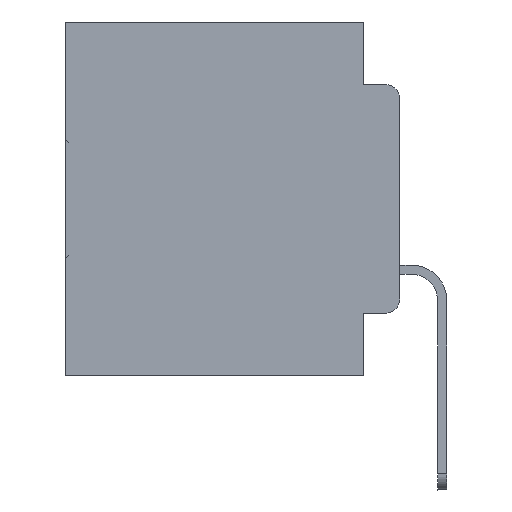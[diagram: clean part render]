
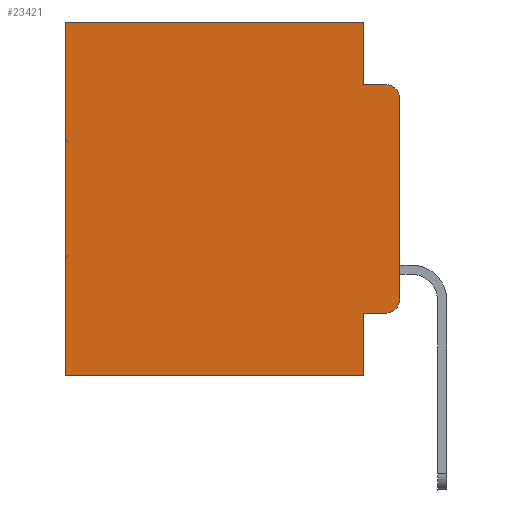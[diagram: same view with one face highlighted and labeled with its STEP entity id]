
A CAD part, left-side view. The second image highlights one B-rep face of the part: STEP entity #23421.
In plain terms, the highlighted planar face has unit normal (-1, 0, 0).
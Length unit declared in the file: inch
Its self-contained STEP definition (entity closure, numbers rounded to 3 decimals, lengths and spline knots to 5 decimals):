
#5 = DIRECTION ( 'NONE',  ( 1., 0., 0. ) ) ;
#20 = EDGE_CURVE ( 'NONE', #6397, #1886, #21172, .T. ) ;
#800 = CARTESIAN_POINT ( 'NONE',  ( 0.298, 0.473, 0. ) ) ;
#909 = VERTEX_POINT ( 'NONE', #26508 ) ;
#1021 = CIRCLE ( 'NONE', #22861, 0.02 ) ;
#1120 = CARTESIAN_POINT ( 'NONE',  ( 0.298, 0.051, -0.4115 ) ) ;
#1125 = VERTEX_POINT ( 'NONE', #22896 ) ;
#1173 = CARTESIAN_POINT ( 'NONE',  ( 0.298, 0.051, 0. ) ) ;
#1886 = VERTEX_POINT ( 'NONE', #12720 ) ;
#1897 = CARTESIAN_POINT ( 'NONE',  ( 0.298, 0.051, -0.0885 ) ) ;
#2144 = AXIS2_PLACEMENT_3D ( 'NONE', #3751, #5, #31906 ) ;
#2297 = DIRECTION ( 'NONE',  ( 0., 0., -1. ) ) ;
#2820 = EDGE_CURVE ( 'NONE', #12477, #6620, #18144, .T. ) ;
#2948 = VERTEX_POINT ( 'NONE', #6425 ) ;
#3010 = CARTESIAN_POINT ( 'NONE',  ( 0.298, 0.051, 0. ) ) ;
#3590 = FACE_OUTER_BOUND ( 'NONE', #11234, .T. ) ;
#3751 = CARTESIAN_POINT ( 'NONE',  ( 0.298, 0., 0. ) ) ;
#4427 = CARTESIAN_POINT ( 'NONE',  ( 0.298, 0.051, 0. ) ) ;
#4510 = ORIENTED_EDGE ( 'NONE', *, *, #13917, .T. ) ;
#5622 = ORIENTED_EDGE ( 'NONE', *, *, #18519, .F. ) ;
#5911 = DIRECTION ( 'NONE',  ( 0., 0., -1. ) ) ;
#6081 = ORIENTED_EDGE ( 'NONE', *, *, #21125, .F. ) ;
#6397 = VERTEX_POINT ( 'NONE', #4427 ) ;
#6425 = CARTESIAN_POINT ( 'NONE',  ( 0.298, 0.473, -0.5 ) ) ;
#6620 = VERTEX_POINT ( 'NONE', #25820 ) ;
#6802 = VECTOR ( 'NONE', #19143, 39.37008 ) ;
#7545 = VECTOR ( 'NONE', #28842, 39.37008 ) ;
#8650 = CARTESIAN_POINT ( 'NONE',  ( 0.298, 0., 0. ) ) ;
#8699 = VECTOR ( 'NONE', #30675, 39.37008 ) ;
#9064 = LINE ( 'NONE', #1897, #6802 ) ;
#9298 = CARTESIAN_POINT ( 'NONE',  ( 0.298, 0., -0.5 ) ) ;
#10515 = DIRECTION ( 'NONE',  ( 0., 0., -1. ) ) ;
#10802 = CARTESIAN_POINT ( 'NONE',  ( 0.298, 0.02, -0.3915 ) ) ;
#11234 = EDGE_LOOP ( 'NONE', ( #30534, #20352, #5622, #6081, #18322, #4510, #27041, #26070, #20592, #11440 ) ) ;
#11243 = EDGE_CURVE ( 'NONE', #18020, #28091, #24690, .T. ) ;
#11393 = CARTESIAN_POINT ( 'NONE',  ( 0.298, 0.02, -0.4115 ) ) ;
#11440 = ORIENTED_EDGE ( 'NONE', *, *, #11837, .T. ) ;
#11691 = VECTOR ( 'NONE', #19012, 39.37008 ) ;
#11837 = EDGE_CURVE ( 'NONE', #28091, #6620, #18080, .T. ) ;
#11838 = CARTESIAN_POINT ( 'NONE',  ( 0.298, 0.051, -0.4115 ) ) ;
#11879 = VERTEX_POINT ( 'NONE', #25911 ) ;
#12144 = VECTOR ( 'NONE', #10515, 39.37008 ) ;
#12477 = VERTEX_POINT ( 'NONE', #21923 ) ;
#12698 = LINE ( 'NONE', #800, #22877 ) ;
#12720 = CARTESIAN_POINT ( 'NONE',  ( 0.298, 0.473, 0. ) ) ;
#13520 = PLANE ( 'NONE',  #2144 ) ;
#13917 = EDGE_CURVE ( 'NONE', #1886, #2948, #12698, .T. ) ;
#14033 = LINE ( 'NONE', #9298, #14795 ) ;
#14795 = VECTOR ( 'NONE', #29005, 39.37008 ) ;
#15482 = AXIS2_PLACEMENT_3D ( 'NONE', #10802, #18277, #5911 ) ;
#17260 = CARTESIAN_POINT ( 'NONE',  ( 0.298, 0.02, -0.1085 ) ) ;
#17596 = EDGE_CURVE ( 'NONE', #12477, #11879, #1021, .T. ) ;
#17700 = VECTOR ( 'NONE', #28203, 39.37008 ) ;
#18020 = VERTEX_POINT ( 'NONE', #1120 ) ;
#18080 = CIRCLE ( 'NONE', #15482, 0.02 ) ;
#18144 = LINE ( 'NONE', #25629, #8699 ) ;
#18268 = LINE ( 'NONE', #1173, #17700 ) ;
#18277 = DIRECTION ( 'NONE',  ( -1., 0., 0. ) ) ;
#18322 = ORIENTED_EDGE ( 'NONE', *, *, #20, .T. ) ;
#18519 = EDGE_CURVE ( 'NONE', #1125, #11879, #9064, .T. ) ;
#19012 = DIRECTION ( 'NONE',  ( 0., -1., 0. ) ) ;
#19143 = DIRECTION ( 'NONE',  ( 0., -1., 0. ) ) ;
#19222 = DIRECTION ( 'NONE',  ( -1., 0., 0. ) ) ;
#20352 = ORIENTED_EDGE ( 'NONE', *, *, #17596, .T. ) ;
#20592 = ORIENTED_EDGE ( 'NONE', *, *, #11243, .T. ) ;
#21125 = EDGE_CURVE ( 'NONE', #6397, #1125, #25325, .T. ) ;
#21172 = LINE ( 'NONE', #8650, #7545 ) ;
#21923 = CARTESIAN_POINT ( 'NONE',  ( 0.298, 0., -0.1085 ) ) ;
#22861 = AXIS2_PLACEMENT_3D ( 'NONE', #17260, #19222, #2297 ) ;
#22877 = VECTOR ( 'NONE', #22922, 39.37008 ) ;
#22896 = CARTESIAN_POINT ( 'NONE',  ( 0.298, 0.051, -0.0885 ) ) ;
#22922 = DIRECTION ( 'NONE',  ( 0., 0., -1. ) ) ;
#23421 = ADVANCED_FACE ( 'NONE', ( #3590 ), #13520, .F. ) ;
#24690 = LINE ( 'NONE', #11838, #11691 ) ;
#25325 = LINE ( 'NONE', #3010, #12144 ) ;
#25629 = CARTESIAN_POINT ( 'NONE',  ( 0.298, 0., 0. ) ) ;
#25820 = CARTESIAN_POINT ( 'NONE',  ( 0.298, 0., -0.3915 ) ) ;
#25911 = CARTESIAN_POINT ( 'NONE',  ( 0.298, 0.02, -0.0885 ) ) ;
#26070 = ORIENTED_EDGE ( 'NONE', *, *, #28660, .F. ) ;
#26508 = CARTESIAN_POINT ( 'NONE',  ( 0.298, 0.051, -0.5 ) ) ;
#26654 = EDGE_CURVE ( 'NONE', #909, #2948, #14033, .T. ) ;
#27041 = ORIENTED_EDGE ( 'NONE', *, *, #26654, .F. ) ;
#28091 = VERTEX_POINT ( 'NONE', #11393 ) ;
#28203 = DIRECTION ( 'NONE',  ( 0., 0., -1. ) ) ;
#28660 = EDGE_CURVE ( 'NONE', #18020, #909, #18268, .T. ) ;
#28842 = DIRECTION ( 'NONE',  ( 0., 1., 0. ) ) ;
#29005 = DIRECTION ( 'NONE',  ( 0., 1., 0. ) ) ;
#30534 = ORIENTED_EDGE ( 'NONE', *, *, #2820, .F. ) ;
#30675 = DIRECTION ( 'NONE',  ( 0., 0., -1. ) ) ;
#31906 = DIRECTION ( 'NONE',  ( 0., 0., -1. ) ) ;
